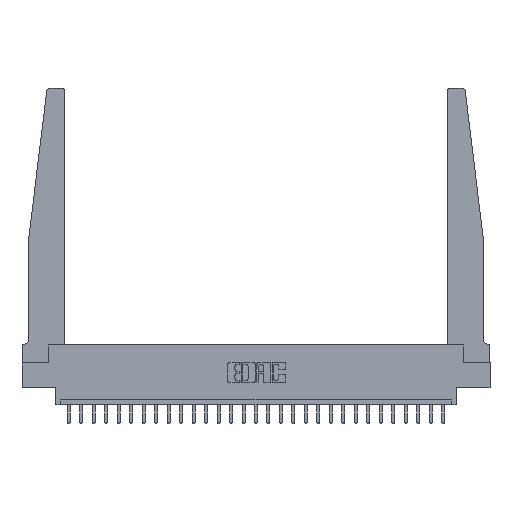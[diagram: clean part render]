
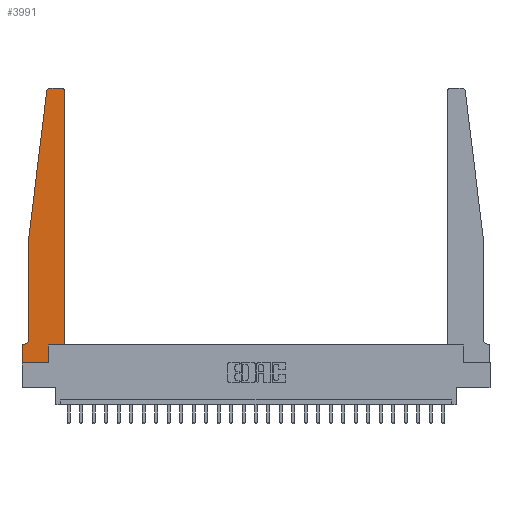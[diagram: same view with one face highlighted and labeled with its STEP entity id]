
A CAD part, top view. The second image highlights one B-rep face of the part: STEP entity #3991.
In plain terms, the highlighted planar face has unit normal (0, 0, 1).
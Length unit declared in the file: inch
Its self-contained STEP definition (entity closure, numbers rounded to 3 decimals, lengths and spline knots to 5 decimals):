
#105 = VERTEX_POINT ( 'NONE', #17992 ) ;
#155 = EDGE_CURVE ( 'NONE', #3024, #16908, #24994, .T. ) ;
#209 = CIRCLE ( 'NONE', #25579, 0.05 ) ;
#397 = CARTESIAN_POINT ( 'NONE',  ( 0.2605, 0.18, 0.37 ) ) ;
#509 = CARTESIAN_POINT ( 'NONE',  ( 0.25, 2.75, 0.37 ) ) ;
#783 = CARTESIAN_POINT ( 'NONE',  ( 0.015, 0.2375, 0.37 ) ) ;
#1016 = EDGE_CURVE ( 'NONE', #21098, #7520, #4427, .T. ) ;
#1181 = CARTESIAN_POINT ( 'NONE',  ( 0., 0., 0.37 ) ) ;
#2135 = EDGE_CURVE ( 'NONE', #18612, #22533, #14504, .T. ) ;
#2239 = AXIS2_PLACEMENT_3D ( 'NONE', #3065, #4939, #20828 ) ;
#2320 = CARTESIAN_POINT ( 'NONE',  ( 0., 0., 0.37 ) ) ;
#2709 = DIRECTION ( 'NONE',  ( 0., 1., 0. ) ) ;
#2766 = CARTESIAN_POINT ( 'NONE',  ( 0.2605, 0., 0.37 ) ) ;
#2969 = ORIENTED_EDGE ( 'NONE', *, *, #1016, .T. ) ;
#3024 = VERTEX_POINT ( 'NONE', #24613 ) ;
#3065 = CARTESIAN_POINT ( 'NONE',  ( 0.27653, 2.72, 0.37 ) ) ;
#3826 = VECTOR ( 'NONE', #16343, 39.37008 ) ;
#3991 = ADVANCED_FACE ( 'NONE', ( #22930 ), #18945, .T. ) ;
#4093 = VECTOR ( 'NONE', #2709, 39.37008 ) ;
#4191 = CARTESIAN_POINT ( 'NONE',  ( 0.065, 1.25, 0.37 ) ) ;
#4427 = LINE ( 'NONE', #20583, #21476 ) ;
#4554 = DIRECTION ( 'NONE',  ( -1., 0., 0. ) ) ;
#4939 = DIRECTION ( 'NONE',  ( 0., 0., 1. ) ) ;
#4994 = VERTEX_POINT ( 'NONE', #7072 ) ;
#5281 = ORIENTED_EDGE ( 'NONE', *, *, #19430, .T. ) ;
#5739 = CARTESIAN_POINT ( 'NONE',  ( 0.2605, 0.18, 0.37 ) ) ;
#6266 = VECTOR ( 'NONE', #6968, 39.37008 ) ;
#6399 = CARTESIAN_POINT ( 'NONE',  ( 0.065, 1.25, 0.37 ) ) ;
#6611 = DIRECTION ( 'NONE',  ( 0., 1., 0. ) ) ;
#6968 = DIRECTION ( 'NONE',  ( -1., 0., 0. ) ) ;
#7003 = ORIENTED_EDGE ( 'NONE', *, *, #16203, .T. ) ;
#7072 = CARTESIAN_POINT ( 'NONE',  ( 0.425, 2.72, 0.37 ) ) ;
#7076 = ORIENTED_EDGE ( 'NONE', *, *, #9878, .T. ) ;
#7093 = VERTEX_POINT ( 'NONE', #2320 ) ;
#7520 = VERTEX_POINT ( 'NONE', #14964 ) ;
#8526 = CARTESIAN_POINT ( 'NONE',  ( 0.065, 0.2375, 0.37 ) ) ;
#8534 = DIRECTION ( 'NONE',  ( -0.122, -0.992, 0. ) ) ;
#8772 = DIRECTION ( 'NONE',  ( 1., 0., 0. ) ) ;
#8789 = LINE ( 'NONE', #24949, #4093 ) ;
#8877 = CARTESIAN_POINT ( 'NONE',  ( 0., 0.1875, 0.37 ) ) ;
#9065 = ORIENTED_EDGE ( 'NONE', *, *, #16711, .T. ) ;
#9497 = CARTESIAN_POINT ( 'NONE',  ( 0.015, 0.1875, 0.37 ) ) ;
#9529 = DIRECTION ( 'NONE',  ( 1., 0., 0. ) ) ;
#9878 = EDGE_CURVE ( 'NONE', #105, #19628, #24794, .T. ) ;
#11212 = VERTEX_POINT ( 'NONE', #23299 ) ;
#11300 = CARTESIAN_POINT ( 'NONE',  ( 0.395, 2.72, 0.37 ) ) ;
#11518 = LINE ( 'NONE', #1181, #21043 ) ;
#11905 = ORIENTED_EDGE ( 'NONE', *, *, #13688, .T. ) ;
#11977 = ORIENTED_EDGE ( 'NONE', *, *, #2135, .T. ) ;
#12064 = DIRECTION ( 'NONE',  ( 0., -1., 0. ) ) ;
#13688 = EDGE_CURVE ( 'NONE', #4994, #3024, #17479, .T. ) ;
#13745 = VECTOR ( 'NONE', #6611, 39.37008 ) ;
#14008 = ORIENTED_EDGE ( 'NONE', *, *, #21293, .T. ) ;
#14504 = LINE ( 'NONE', #20972, #20687 ) ;
#14603 = DIRECTION ( 'NONE',  ( 0., 0., 1. ) ) ;
#14964 = CARTESIAN_POINT ( 'NONE',  ( 0., 0.1875, 0.37 ) ) ;
#15503 = ORIENTED_EDGE ( 'NONE', *, *, #19185, .T. ) ;
#15767 = ORIENTED_EDGE ( 'NONE', *, *, #21906, .T. ) ;
#16203 = EDGE_CURVE ( 'NONE', #11212, #105, #24693, .T. ) ;
#16231 = AXIS2_PLACEMENT_3D ( 'NONE', #11300, #23212, #25707 ) ;
#16343 = DIRECTION ( 'NONE',  ( 0., -1., 0. ) ) ;
#16711 = EDGE_CURVE ( 'NONE', #16908, #11212, #17874, .T. ) ;
#16908 = VERTEX_POINT ( 'NONE', #20380 ) ;
#17479 = CIRCLE ( 'NONE', #16231, 0.03 ) ;
#17874 = CIRCLE ( 'NONE', #2239, 0.03 ) ;
#17992 = CARTESIAN_POINT ( 'NONE',  ( 0.065, 1.25, 0.37 ) ) ;
#18080 = CARTESIAN_POINT ( 'NONE',  ( 0.425, 0.18, 0.37 ) ) ;
#18090 = EDGE_LOOP ( 'NONE', ( #19711, #9065, #7003, #7076, #5281, #2969, #23979, #15767, #15503, #11977, #14008, #11905 ) ) ;
#18535 = LINE ( 'NONE', #397, #13745 ) ;
#18612 = VERTEX_POINT ( 'NONE', #5739 ) ;
#18768 = VECTOR ( 'NONE', #8534, 39.37008 ) ;
#18945 = PLANE ( 'NONE',  #24880 ) ;
#19185 = EDGE_CURVE ( 'NONE', #19421, #18612, #18535, .T. ) ;
#19421 = VERTEX_POINT ( 'NONE', #2766 ) ;
#19430 = EDGE_CURVE ( 'NONE', #19628, #21098, #209, .T. ) ;
#19628 = VERTEX_POINT ( 'NONE', #8526 ) ;
#19711 = ORIENTED_EDGE ( 'NONE', *, *, #155, .T. ) ;
#20276 = CARTESIAN_POINT ( 'NONE',  ( 0., 0., 0.37 ) ) ;
#20380 = CARTESIAN_POINT ( 'NONE',  ( 0.27653, 2.75, 0.37 ) ) ;
#20583 = CARTESIAN_POINT ( 'NONE',  ( 0.065, 0.1875, 0.37 ) ) ;
#20687 = VECTOR ( 'NONE', #8772, 39.37008 ) ;
#20828 = DIRECTION ( 'NONE',  ( 1., 0., 0. ) ) ;
#20972 = CARTESIAN_POINT ( 'NONE',  ( 0.425, 0.18, 0.37 ) ) ;
#21021 = VECTOR ( 'NONE', #12064, 39.37008 ) ;
#21043 = VECTOR ( 'NONE', #9529, 39.37008 ) ;
#21046 = DIRECTION ( 'NONE',  ( 0., 0., -1. ) ) ;
#21098 = VERTEX_POINT ( 'NONE', #9497 ) ;
#21293 = EDGE_CURVE ( 'NONE', #22533, #4994, #8789, .T. ) ;
#21476 = VECTOR ( 'NONE', #4554, 39.37008 ) ;
#21569 = EDGE_CURVE ( 'NONE', #7520, #7093, #22265, .T. ) ;
#21906 = EDGE_CURVE ( 'NONE', #7093, #19421, #11518, .T. ) ;
#22265 = LINE ( 'NONE', #20276, #21021 ) ;
#22533 = VERTEX_POINT ( 'NONE', #18080 ) ;
#22671 = DIRECTION ( 'NONE',  ( 1., 0., 0. ) ) ;
#22930 = FACE_OUTER_BOUND ( 'NONE', #18090, .T. ) ;
#23212 = DIRECTION ( 'NONE',  ( 0., 0., 1. ) ) ;
#23299 = CARTESIAN_POINT ( 'NONE',  ( 0.24675, 2.72367, 0.37 ) ) ;
#23979 = ORIENTED_EDGE ( 'NONE', *, *, #21569, .T. ) ;
#24613 = CARTESIAN_POINT ( 'NONE',  ( 0.395, 2.75, 0.37 ) ) ;
#24693 = LINE ( 'NONE', #4191, #18768 ) ;
#24794 = LINE ( 'NONE', #6399, #3826 ) ;
#24880 = AXIS2_PLACEMENT_3D ( 'NONE', #8877, #14603, #22671 ) ;
#24949 = CARTESIAN_POINT ( 'NONE',  ( 0.425, 0.18, 0.37 ) ) ;
#24994 = LINE ( 'NONE', #509, #6266 ) ;
#25005 = DIRECTION ( 'NONE',  ( -1., 0., 0. ) ) ;
#25579 = AXIS2_PLACEMENT_3D ( 'NONE', #783, #21046, #25005 ) ;
#25707 = DIRECTION ( 'NONE',  ( 1., 0., 0. ) ) ;
